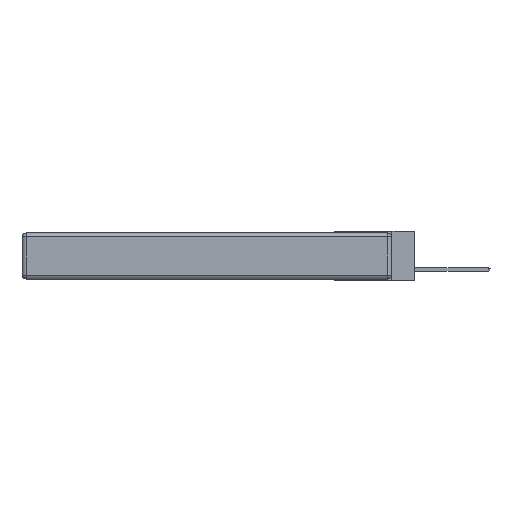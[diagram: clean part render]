
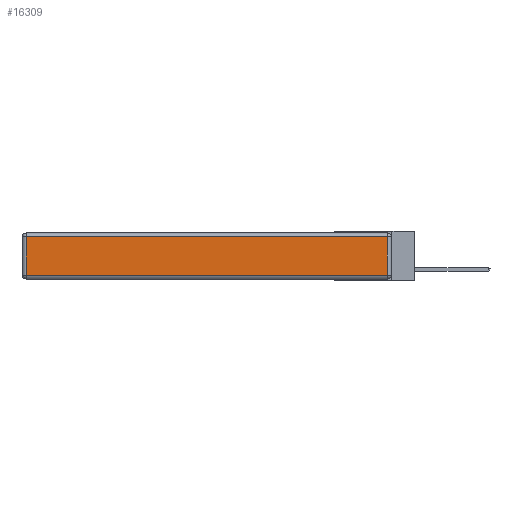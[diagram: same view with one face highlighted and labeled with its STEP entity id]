
A CAD part, left-side view. The second image highlights one B-rep face of the part: STEP entity #16309.
In plain terms, the highlighted planar face has unit normal (-1, 0, 0).
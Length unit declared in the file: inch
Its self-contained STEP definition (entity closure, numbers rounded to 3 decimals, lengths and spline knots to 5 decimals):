
#580 = VERTEX_POINT ( 'NONE', #3790 ) ;
#2365 = ORIENTED_EDGE ( 'NONE', *, *, #12881, .T. ) ;
#2423 = PLANE ( 'NONE',  #19732 ) ;
#3790 = CARTESIAN_POINT ( 'NONE',  ( 0., 2.72, -0.313 ) ) ;
#4009 = CARTESIAN_POINT ( 'NONE',  ( 0., 2.72, -0.343 ) ) ;
#4225 = DIRECTION ( 'NONE',  ( 0., 0., 1. ) ) ;
#5707 = DIRECTION ( 'NONE',  ( -1., 0., 0. ) ) ;
#7052 = CARTESIAN_POINT ( 'NONE',  ( 0., 0., -0.313 ) ) ;
#7553 = EDGE_CURVE ( 'NONE', #580, #8403, #14455, .T. ) ;
#8403 = VERTEX_POINT ( 'NONE', #13007 ) ;
#8615 = EDGE_CURVE ( 'NONE', #13474, #11293, #10634, .T. ) ;
#9373 = CARTESIAN_POINT ( 'NONE',  ( 0., 0.03, -0.343 ) ) ;
#10070 = DIRECTION ( 'NONE',  ( 0., 1., 0. ) ) ;
#10634 = LINE ( 'NONE', #20120, #11164 ) ;
#10669 = CARTESIAN_POINT ( 'NONE',  ( 0., 2.72, -0.03 ) ) ;
#11164 = VECTOR ( 'NONE', #10070, 39.37008 ) ;
#11293 = VERTEX_POINT ( 'NONE', #10669 ) ;
#12845 = CARTESIAN_POINT ( 'NONE',  ( 0., 0., -0.343 ) ) ;
#12881 = EDGE_CURVE ( 'NONE', #11293, #580, #22301, .T. ) ;
#12973 = EDGE_CURVE ( 'NONE', #8403, #13474, #14117, .T. ) ;
#13007 = CARTESIAN_POINT ( 'NONE',  ( 0., 0.03, -0.313 ) ) ;
#13474 = VERTEX_POINT ( 'NONE', #22233 ) ;
#13496 = FACE_OUTER_BOUND ( 'NONE', #17151, .T. ) ;
#14035 = DIRECTION ( 'NONE',  ( 0., -1., 0. ) ) ;
#14117 = LINE ( 'NONE', #9373, #21738 ) ;
#14455 = LINE ( 'NONE', #7052, #14707 ) ;
#14707 = VECTOR ( 'NONE', #14035, 39.37008 ) ;
#16285 = ORIENTED_EDGE ( 'NONE', *, *, #8615, .T. ) ;
#16309 = ADVANCED_FACE ( 'NONE', ( #13496 ), #2423, .T. ) ;
#17151 = EDGE_LOOP ( 'NONE', ( #19356, #20472, #16285, #2365 ) ) ;
#17664 = VECTOR ( 'NONE', #19576, 39.37008 ) ;
#18063 = DIRECTION ( 'NONE',  ( 0., 0., 1. ) ) ;
#19356 = ORIENTED_EDGE ( 'NONE', *, *, #7553, .T. ) ;
#19576 = DIRECTION ( 'NONE',  ( 0., 0., -1. ) ) ;
#19732 = AXIS2_PLACEMENT_3D ( 'NONE', #12845, #5707, #18063 ) ;
#20120 = CARTESIAN_POINT ( 'NONE',  ( 0., 2.75, -0.03 ) ) ;
#20472 = ORIENTED_EDGE ( 'NONE', *, *, #12973, .T. ) ;
#21738 = VECTOR ( 'NONE', #4225, 39.37008 ) ;
#22233 = CARTESIAN_POINT ( 'NONE',  ( 0., 0.03, -0.03 ) ) ;
#22301 = LINE ( 'NONE', #4009, #17664 ) ;
